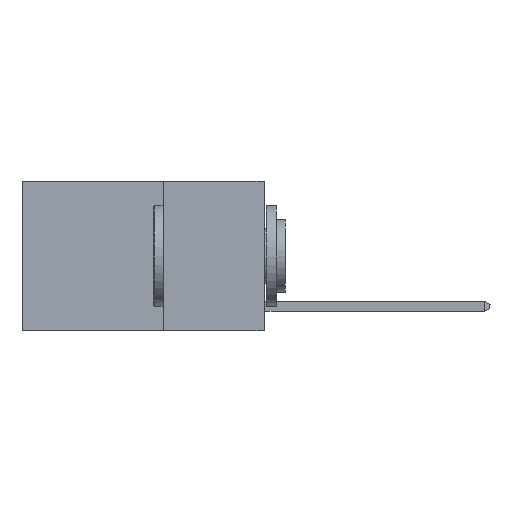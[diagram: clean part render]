
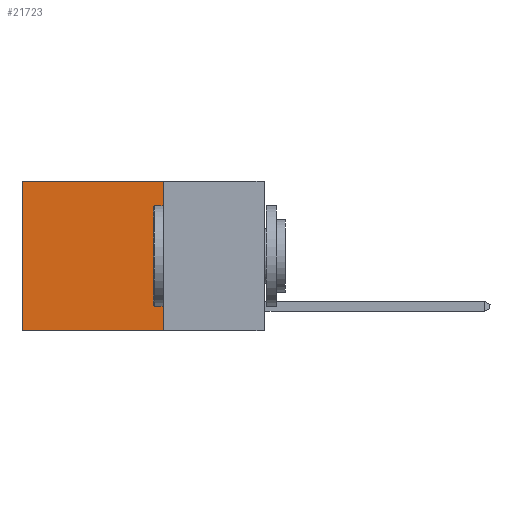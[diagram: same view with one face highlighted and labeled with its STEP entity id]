
A CAD part, left-side view. The second image highlights one B-rep face of the part: STEP entity #21723.
In plain terms, the highlighted planar face has unit normal (-1, 0, 0).
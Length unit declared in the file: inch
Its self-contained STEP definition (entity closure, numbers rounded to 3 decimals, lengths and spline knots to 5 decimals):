
#360 = LINE ( 'NONE', #19577, #11552 ) ;
#812 = DIRECTION ( 'NONE',  ( 0., 0., -1. ) ) ;
#916 = CARTESIAN_POINT ( 'NONE',  ( 0.2625, 0.25, -0.37 ) ) ;
#1671 = CARTESIAN_POINT ( 'NONE',  ( 0.2625, 0.25, 0. ) ) ;
#4456 = EDGE_CURVE ( 'NONE', #21130, #11590, #360, .T. ) ;
#5600 = CARTESIAN_POINT ( 'NONE',  ( 0.2625, 0.25, 0. ) ) ;
#5929 = PLANE ( 'NONE',  #8657 ) ;
#8657 = AXIS2_PLACEMENT_3D ( 'NONE', #23620, #10428, #25874 ) ;
#10012 = DIRECTION ( 'NONE',  ( 0., 1., 0. ) ) ;
#10428 = DIRECTION ( 'NONE',  ( 1., 0., 0. ) ) ;
#10962 = VERTEX_POINT ( 'NONE', #21835 ) ;
#11552 = VECTOR ( 'NONE', #15251, 39.37008 ) ;
#11590 = VERTEX_POINT ( 'NONE', #19697 ) ;
#12879 = EDGE_CURVE ( 'NONE', #13294, #10962, #27480, .T. ) ;
#13294 = VERTEX_POINT ( 'NONE', #26653 ) ;
#13729 = FACE_OUTER_BOUND ( 'NONE', #17507, .T. ) ;
#14198 = ORIENTED_EDGE ( 'NONE', *, *, #15212, .T. ) ;
#14254 = DIRECTION ( 'NONE',  ( 0., 1., 0. ) ) ;
#14378 = VECTOR ( 'NONE', #10012, 39.37008 ) ;
#15089 = VECTOR ( 'NONE', #812, 39.37008 ) ;
#15212 = EDGE_CURVE ( 'NONE', #21130, #13294, #26126, .T. ) ;
#15251 = DIRECTION ( 'NONE',  ( 0., 0., -1. ) ) ;
#17507 = EDGE_LOOP ( 'NONE', ( #26542, #19784, #25847, #14198 ) ) ;
#18170 = VECTOR ( 'NONE', #14254, 39.37008 ) ;
#19577 = CARTESIAN_POINT ( 'NONE',  ( 0.2625, 0.25, 0. ) ) ;
#19697 = CARTESIAN_POINT ( 'NONE',  ( 0.2625, 0.25, -0.37 ) ) ;
#19784 = ORIENTED_EDGE ( 'NONE', *, *, #22170, .F. ) ;
#21130 = VERTEX_POINT ( 'NONE', #1671 ) ;
#21723 = ADVANCED_FACE ( 'NONE', ( #13729 ), #5929, .F. ) ;
#21835 = CARTESIAN_POINT ( 'NONE',  ( 0.2625, 0.6, -0.37 ) ) ;
#22170 = EDGE_CURVE ( 'NONE', #11590, #10962, #24054, .T. ) ;
#23620 = CARTESIAN_POINT ( 'NONE',  ( 0.2625, 0.25, 0. ) ) ;
#24054 = LINE ( 'NONE', #916, #18170 ) ;
#25847 = ORIENTED_EDGE ( 'NONE', *, *, #4456, .F. ) ;
#25874 = DIRECTION ( 'NONE',  ( 0., 0., -1. ) ) ;
#26126 = LINE ( 'NONE', #5600, #14378 ) ;
#26542 = ORIENTED_EDGE ( 'NONE', *, *, #12879, .T. ) ;
#26653 = CARTESIAN_POINT ( 'NONE',  ( 0.2625, 0.6, 0. ) ) ;
#27354 = CARTESIAN_POINT ( 'NONE',  ( 0.2625, 0.6, 0. ) ) ;
#27480 = LINE ( 'NONE', #27354, #15089 ) ;
